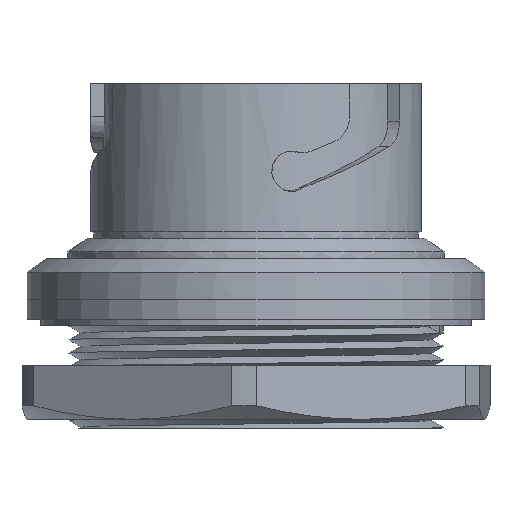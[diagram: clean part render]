
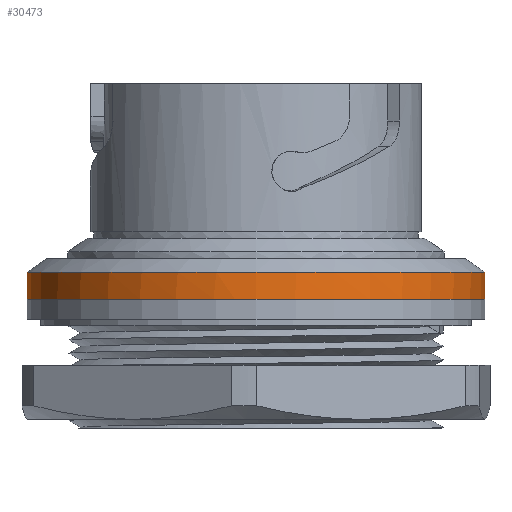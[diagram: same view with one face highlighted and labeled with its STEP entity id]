
A CAD part, front view. The second image highlights one B-rep face of the part: STEP entity #30473.
In plain terms, the highlighted cylindrical face has radius 17 mm (diameter 34 mm), a partial arc.
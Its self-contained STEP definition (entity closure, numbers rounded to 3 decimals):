
#2205 = CARTESIAN_POINT ( 'NONE',  ( -16., -1.113, 17. ) ) ;
#2971 = CARTESIAN_POINT ( 'NONE',  ( -16., -14.753, 8.52 ) ) ;
#3572 = B_SPLINE_CURVE_WITH_KNOTS ( 'NONE', 3,
 ( #32580, #2205, #36891, #32824, #17501, #33066, #21577, #13948, #49359, #50117, #18766, #2971, #7045, #34071, #14695, #22585, #10372, #41714 ),
 .UNSPECIFIED., .F., .F.,
 ( 4, 2, 2, 2, 2, 2, 2, 2, 4 ),
 ( 0.5, 0.563, 0.625, 0.688, 0.75, 0.813, 0.875, 0.938, 1. ),
 .UNSPECIFIED. ) ;
#4761 = ORIENTED_EDGE ( 'NONE', *, *, #48957, .T. ) ;
#5665 = EDGE_CURVE ( 'NONE', #10433, #6835, #41083, .T. ) ;
#6171 = DIRECTION ( 'NONE',  ( 1., 0., 0. ) ) ;
#6835 = VERTEX_POINT ( 'NONE', #34743 ) ;
#7045 = CARTESIAN_POINT ( 'NONE',  ( -16., -15.28, 7.534 ) ) ;
#7310 = CARTESIAN_POINT ( 'NONE',  ( -16., -13.517, -10.37 ) ) ;
#7557 = CARTESIAN_POINT ( 'NONE',  ( -16., -15.28, -7.534 ) ) ;
#7801 = CARTESIAN_POINT ( 'NONE',  ( -16., -17., -1.113 ) ) ;
#8058 = CARTESIAN_POINT ( 'NONE',  ( -16., -17., 0. ) ) ;
#8587 = ORIENTED_EDGE ( 'NONE', *, *, #5665, .T. ) ;
#8710 = EDGE_CURVE ( 'NONE', #44077, #41498, #25723, .T. ) ;
#9809 = DIRECTION ( 'NONE',  ( 1., 0., 0. ) ) ;
#10372 = CARTESIAN_POINT ( 'NONE',  ( -16., -17., 1.113 ) ) ;
#10433 = VERTEX_POINT ( 'NONE', #36307 ) ;
#10882 = CARTESIAN_POINT ( 'NONE',  ( -16., -1.113, -17. ) ) ;
#11964 = DIRECTION ( 'NONE',  ( -1., 0., 0. ) ) ;
#13948 = CARTESIAN_POINT ( 'NONE',  ( -16., -10.37, 13.517 ) ) ;
#14695 = CARTESIAN_POINT ( 'NONE',  ( -16., -16.456, 4.408 ) ) ;
#14843 = ORIENTED_EDGE ( 'NONE', *, *, #19258, .T. ) ;
#14943 = CARTESIAN_POINT ( 'NONE',  ( -16., -5.478, -16.132 ) ) ;
#15461 = CARTESIAN_POINT ( 'NONE',  ( -16., -7.534, -15.28 ) ) ;
#15705 = CARTESIAN_POINT ( 'NONE',  ( -16., -16.89, -2.225 ) ) ;
#17444 = CYLINDRICAL_SURFACE ( 'NONE', #30189, 17. ) ;
#17501 = CARTESIAN_POINT ( 'NONE',  ( -16., -5.478, 16.132 ) ) ;
#18271 = VECTOR ( 'NONE', #6171, 1000. ) ;
#18766 = CARTESIAN_POINT ( 'NONE',  ( -16., -13.517, 10.37 ) ) ;
#19258 = EDGE_CURVE ( 'NONE', #25266, #10433, #19606, .T. ) ;
#19263 = CARTESIAN_POINT ( 'NONE',  ( -16., -16.456, -4.408 ) ) ;
#19318 = CIRCLE ( 'NONE', #26674, 17. ) ;
#19606 = B_SPLINE_CURVE_WITH_KNOTS ( 'NONE', 3,
 ( #8058, #7801, #15705, #19263, #46297, #7557, #46553, #7310, #42988, #27432, #34328, #45787, #15461, #14943, #22846, #31024, #10882, #38162 ),
 .UNSPECIFIED., .F., .F.,
 ( 4, 2, 2, 2, 2, 2, 2, 2, 4 ),
 ( 0., 0.062, 0.125, 0.187, 0.25, 0.312, 0.375, 0.437, 0.5 ),
 .UNSPECIFIED. ) ;
#19840 = DIRECTION ( 'NONE',  ( 0., 0., -1. ) ) ;
#21577 = CARTESIAN_POINT ( 'NONE',  ( -16., -8.52, 14.753 ) ) ;
#22585 = CARTESIAN_POINT ( 'NONE',  ( -16., -16.89, 2.225 ) ) ;
#22846 = CARTESIAN_POINT ( 'NONE',  ( -16., -4.408, -16.456 ) ) ;
#23078 = ORIENTED_EDGE ( 'NONE', *, *, #46748, .T. ) ;
#25266 = VERTEX_POINT ( 'NONE', #44717 ) ;
#25723 = LINE ( 'NONE', #37958, #44371 ) ;
#26674 = AXIS2_PLACEMENT_3D ( 'NONE', #47123, #11964, #19840 ) ;
#27432 = CARTESIAN_POINT ( 'NONE',  ( -16., -11.234, -12.808 ) ) ;
#29493 = CARTESIAN_POINT ( 'NONE',  ( -16., 0., 17. ) ) ;
#30189 = AXIS2_PLACEMENT_3D ( 'NONE', #48546, #9809, #40900 ) ;
#30473 = ADVANCED_FACE ( 'NONE', ( #44719 ), #17444, .T. ) ;
#31024 = CARTESIAN_POINT ( 'NONE',  ( -16., -2.225, -16.89 ) ) ;
#32580 = CARTESIAN_POINT ( 'NONE',  ( -16., 0., 17. ) ) ;
#32824 = CARTESIAN_POINT ( 'NONE',  ( -16., -4.408, 16.456 ) ) ;
#33066 = CARTESIAN_POINT ( 'NONE',  ( -16., -7.534, 15.28 ) ) ;
#34071 = CARTESIAN_POINT ( 'NONE',  ( -16., -16.132, 5.478 ) ) ;
#34328 = CARTESIAN_POINT ( 'NONE',  ( -16., -10.37, -13.517 ) ) ;
#34743 = CARTESIAN_POINT ( 'NONE',  ( -14., 0., -17. ) ) ;
#36307 = CARTESIAN_POINT ( 'NONE',  ( -16., 0., -17. ) ) ;
#36891 = CARTESIAN_POINT ( 'NONE',  ( -16., -2.225, 16.89 ) ) ;
#37958 = CARTESIAN_POINT ( 'NONE',  ( -26.33, 0., 17. ) ) ;
#38162 = CARTESIAN_POINT ( 'NONE',  ( -16., 0., -17. ) ) ;
#40900 = DIRECTION ( 'NONE',  ( 0., 0., -1. ) ) ;
#41083 = LINE ( 'NONE', #41342, #18271 ) ;
#41274 = DIRECTION ( 'NONE',  ( 1., 0., 0. ) ) ;
#41342 = CARTESIAN_POINT ( 'NONE',  ( -26.33, 0., -17. ) ) ;
#41498 = VERTEX_POINT ( 'NONE', #45271 ) ;
#41714 = CARTESIAN_POINT ( 'NONE',  ( -16., -17., 0. ) ) ;
#42988 = CARTESIAN_POINT ( 'NONE',  ( -16., -12.808, -11.234 ) ) ;
#43973 = EDGE_LOOP ( 'NONE', ( #48067, #4761, #14843, #8587, #23078 ) ) ;
#44077 = VERTEX_POINT ( 'NONE', #29493 ) ;
#44371 = VECTOR ( 'NONE', #41274, 1000. ) ;
#44717 = CARTESIAN_POINT ( 'NONE',  ( -16., -17., 0. ) ) ;
#44719 = FACE_OUTER_BOUND ( 'NONE', #43973, .T. ) ;
#45271 = CARTESIAN_POINT ( 'NONE',  ( -14., 0., 17. ) ) ;
#45787 = CARTESIAN_POINT ( 'NONE',  ( -16., -8.52, -14.753 ) ) ;
#46297 = CARTESIAN_POINT ( 'NONE',  ( -16., -16.132, -5.478 ) ) ;
#46553 = CARTESIAN_POINT ( 'NONE',  ( -16., -14.753, -8.52 ) ) ;
#46748 = EDGE_CURVE ( 'NONE', #6835, #41498, #19318, .T. ) ;
#47123 = CARTESIAN_POINT ( 'NONE',  ( -14., 0., 0. ) ) ;
#48067 = ORIENTED_EDGE ( 'NONE', *, *, #8710, .F. ) ;
#48546 = CARTESIAN_POINT ( 'NONE',  ( -26.33, 0., 0. ) ) ;
#48957 = EDGE_CURVE ( 'NONE', #44077, #25266, #3572, .T. ) ;
#49359 = CARTESIAN_POINT ( 'NONE',  ( -16., -11.234, 12.808 ) ) ;
#50117 = CARTESIAN_POINT ( 'NONE',  ( -16., -12.808, 11.234 ) ) ;
